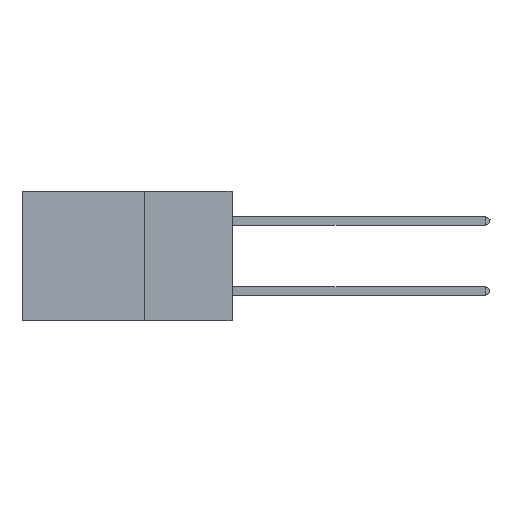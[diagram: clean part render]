
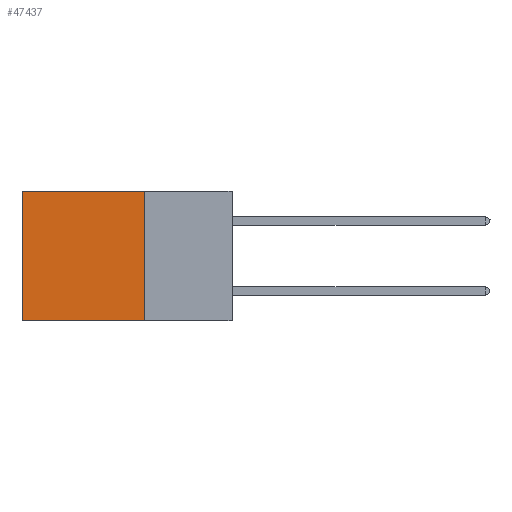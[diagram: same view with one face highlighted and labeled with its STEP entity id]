
A CAD part, left-side view. The second image highlights one B-rep face of the part: STEP entity #47437.
In plain terms, the highlighted planar face has unit normal (-1, 0, 0).
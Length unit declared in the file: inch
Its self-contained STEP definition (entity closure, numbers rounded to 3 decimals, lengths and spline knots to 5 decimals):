
#415 = PLANE ( 'NONE',  #38856 ) ;
#1208 = CARTESIAN_POINT ( 'NONE',  ( 0.2875, 0.6, 0. ) ) ;
#3143 = LINE ( 'NONE', #21921, #42694 ) ;
#4343 = ORIENTED_EDGE ( 'NONE', *, *, #29778, .F. ) ;
#4693 = DIRECTION ( 'NONE',  ( 0., 0., -1. ) ) ;
#4919 = EDGE_CURVE ( 'NONE', #41512, #38148, #17465, .T. ) ;
#5338 = DIRECTION ( 'NONE',  ( 1., 0., 0. ) ) ;
#5551 = ORIENTED_EDGE ( 'NONE', *, *, #4919, .F. ) ;
#6045 = EDGE_CURVE ( 'NONE', #41512, #48364, #3143, .T. ) ;
#6105 = CARTESIAN_POINT ( 'NONE',  ( 0.2875, 0.6, 0. ) ) ;
#9652 = EDGE_LOOP ( 'NONE', ( #28578, #4343, #5551, #38505 ) ) ;
#13277 = VECTOR ( 'NONE', #15741, 39.37008 ) ;
#15741 = DIRECTION ( 'NONE',  ( 0., 1., 0. ) ) ;
#16322 = CARTESIAN_POINT ( 'NONE',  ( 0.2875, 0.6, -0.37 ) ) ;
#17465 = LINE ( 'NONE', #43656, #44924 ) ;
#20065 = CARTESIAN_POINT ( 'NONE',  ( 0.2875, 0.25, -0.37 ) ) ;
#21921 = CARTESIAN_POINT ( 'NONE',  ( 0.2875, 0.25, 0. ) ) ;
#23597 = CARTESIAN_POINT ( 'NONE',  ( 0.2875, 0.25, 0. ) ) ;
#28578 = ORIENTED_EDGE ( 'NONE', *, *, #38575, .T. ) ;
#29573 = CARTESIAN_POINT ( 'NONE',  ( 0.2875, 0.25, 0. ) ) ;
#29778 = EDGE_CURVE ( 'NONE', #38148, #48767, #33756, .T. ) ;
#33756 = LINE ( 'NONE', #38215, #13277 ) ;
#34257 = FACE_OUTER_BOUND ( 'NONE', #9652, .T. ) ;
#35007 = VECTOR ( 'NONE', #4693, 39.37008 ) ;
#38148 = VERTEX_POINT ( 'NONE', #20065 ) ;
#38215 = CARTESIAN_POINT ( 'NONE',  ( 0.2875, 0.25, -0.37 ) ) ;
#38505 = ORIENTED_EDGE ( 'NONE', *, *, #6045, .T. ) ;
#38538 = LINE ( 'NONE', #1208, #35007 ) ;
#38575 = EDGE_CURVE ( 'NONE', #48364, #48767, #38538, .T. ) ;
#38856 = AXIS2_PLACEMENT_3D ( 'NONE', #29573, #5338, #46352 ) ;
#41512 = VERTEX_POINT ( 'NONE', #23597 ) ;
#42694 = VECTOR ( 'NONE', #48374, 39.37008 ) ;
#43656 = CARTESIAN_POINT ( 'NONE',  ( 0.2875, 0.25, 0. ) ) ;
#44924 = VECTOR ( 'NONE', #47610, 39.37008 ) ;
#46352 = DIRECTION ( 'NONE',  ( 0., 0., -1. ) ) ;
#47437 = ADVANCED_FACE ( 'NONE', ( #34257 ), #415, .F. ) ;
#47610 = DIRECTION ( 'NONE',  ( 0., 0., -1. ) ) ;
#48364 = VERTEX_POINT ( 'NONE', #6105 ) ;
#48374 = DIRECTION ( 'NONE',  ( 0., 1., 0. ) ) ;
#48767 = VERTEX_POINT ( 'NONE', #16322 ) ;
